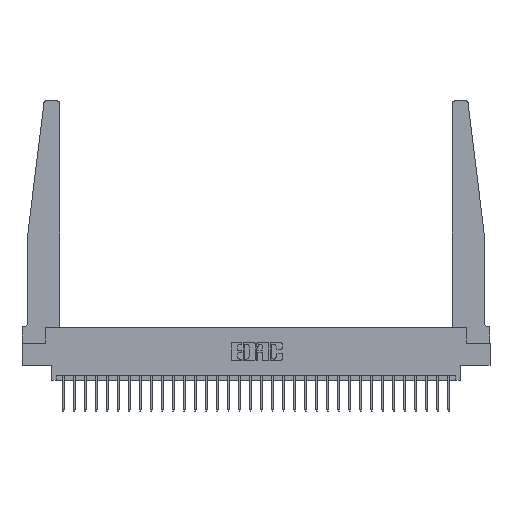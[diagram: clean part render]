
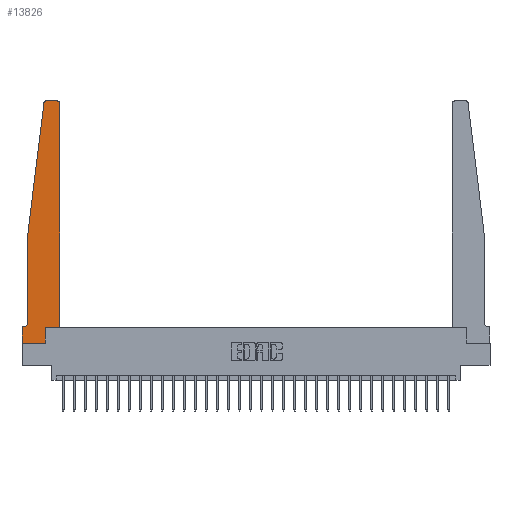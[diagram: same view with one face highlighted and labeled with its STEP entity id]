
A CAD part, top view. The second image highlights one B-rep face of the part: STEP entity #13826.
In plain terms, the highlighted planar face has unit normal (0, 0, 1).
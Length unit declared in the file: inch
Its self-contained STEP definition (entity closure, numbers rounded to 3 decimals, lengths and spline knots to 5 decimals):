
#43 = CARTESIAN_POINT ( 'NONE',  ( 0.015, 0.2375, 0.37 ) ) ;
#174 = EDGE_CURVE ( 'NONE', #27736, #17685, #9732, .T. ) ;
#345 = VERTEX_POINT ( 'NONE', #6715 ) ;
#693 = VECTOR ( 'NONE', #21481, 39.37008 ) ;
#842 = LINE ( 'NONE', #26395, #9476 ) ;
#1305 = DIRECTION ( 'NONE',  ( 0., -1., 0. ) ) ;
#1378 = LINE ( 'NONE', #19375, #19688 ) ;
#1739 = CARTESIAN_POINT ( 'NONE',  ( 0.2605, 0.18, 0.37 ) ) ;
#2248 = VECTOR ( 'NONE', #2393, 39.37008 ) ;
#2262 = CARTESIAN_POINT ( 'NONE',  ( 0.425, 2.72, 0.37 ) ) ;
#2393 = DIRECTION ( 'NONE',  ( -1., 0., 0. ) ) ;
#2428 = DIRECTION ( 'NONE',  ( 0., 0., 1. ) ) ;
#2440 = EDGE_CURVE ( 'NONE', #24999, #11782, #12501, .T. ) ;
#2450 = DIRECTION ( 'NONE',  ( 0., 0., -1. ) ) ;
#2917 = CARTESIAN_POINT ( 'NONE',  ( 0., 0., 0.37 ) ) ;
#2956 = CARTESIAN_POINT ( 'NONE',  ( 0.425, 0.18, 0.37 ) ) ;
#3341 = VECTOR ( 'NONE', #8523, 39.37008 ) ;
#3510 = ORIENTED_EDGE ( 'NONE', *, *, #15467, .T. ) ;
#3787 = CIRCLE ( 'NONE', #24889, 0.03 ) ;
#3964 = EDGE_CURVE ( 'NONE', #28676, #23042, #842, .T. ) ;
#4210 = VERTEX_POINT ( 'NONE', #26830 ) ;
#4221 = VECTOR ( 'NONE', #25952, 39.37008 ) ;
#5036 = DIRECTION ( 'NONE',  ( 0., 1., 0. ) ) ;
#5210 = VERTEX_POINT ( 'NONE', #2956 ) ;
#6071 = ORIENTED_EDGE ( 'NONE', *, *, #174, .T. ) ;
#6579 = ORIENTED_EDGE ( 'NONE', *, *, #21604, .T. ) ;
#6715 = CARTESIAN_POINT ( 'NONE',  ( 0.015, 0.1875, 0.37 ) ) ;
#6956 = DIRECTION ( 'NONE',  ( 1., 0., 0. ) ) ;
#7099 = CARTESIAN_POINT ( 'NONE',  ( 0.065, 1.25, 0.37 ) ) ;
#7100 = EDGE_CURVE ( 'NONE', #17685, #345, #13301, .T. ) ;
#7302 = LINE ( 'NONE', #11934, #28595 ) ;
#7676 = AXIS2_PLACEMENT_3D ( 'NONE', #15869, #11380, #27740 ) ;
#7705 = DIRECTION ( 'NONE',  ( -0.122, -0.992, 0. ) ) ;
#8377 = CIRCLE ( 'NONE', #25133, 0.03 ) ;
#8523 = DIRECTION ( 'NONE',  ( 0., 1., 0. ) ) ;
#8682 = CARTESIAN_POINT ( 'NONE',  ( 0., 0., 0.37 ) ) ;
#8793 = VERTEX_POINT ( 'NONE', #2262 ) ;
#8892 = CARTESIAN_POINT ( 'NONE',  ( 0.065, 0.1875, 0.37 ) ) ;
#9236 = DIRECTION ( 'NONE',  ( -1., 0., 0. ) ) ;
#9476 = VECTOR ( 'NONE', #15243, 39.37008 ) ;
#9732 = LINE ( 'NONE', #14360, #4221 ) ;
#11121 = LINE ( 'NONE', #8892, #2248 ) ;
#11299 = CARTESIAN_POINT ( 'NONE',  ( 0.27653, 2.75, 0.37 ) ) ;
#11380 = DIRECTION ( 'NONE',  ( 0., 0., 1. ) ) ;
#11462 = ORIENTED_EDGE ( 'NONE', *, *, #3964, .T. ) ;
#11782 = VERTEX_POINT ( 'NONE', #11299 ) ;
#11934 = CARTESIAN_POINT ( 'NONE',  ( 0.425, 0.18, 0.37 ) ) ;
#12452 = ORIENTED_EDGE ( 'NONE', *, *, #17511, .T. ) ;
#12501 = LINE ( 'NONE', #21641, #693 ) ;
#13007 = EDGE_CURVE ( 'NONE', #8793, #24999, #3787, .T. ) ;
#13301 = CIRCLE ( 'NONE', #15695, 0.05 ) ;
#13826 = ADVANCED_FACE ( 'NONE', ( #22309 ), #15719, .T. ) ;
#13921 = DIRECTION ( 'NONE',  ( 1., 0., 0. ) ) ;
#14201 = DIRECTION ( 'NONE',  ( 0., 0., 1. ) ) ;
#14360 = CARTESIAN_POINT ( 'NONE',  ( 0.065, 1.25, 0.37 ) ) ;
#15243 = DIRECTION ( 'NONE',  ( 1., 0., 0. ) ) ;
#15252 = LINE ( 'NONE', #8682, #27907 ) ;
#15467 = EDGE_CURVE ( 'NONE', #23042, #4210, #22425, .T. ) ;
#15695 = AXIS2_PLACEMENT_3D ( 'NONE', #43, #2450, #9236 ) ;
#15719 = PLANE ( 'NONE',  #7676 ) ;
#15869 = CARTESIAN_POINT ( 'NONE',  ( 0., 0.1875, 0.37 ) ) ;
#15936 = CARTESIAN_POINT ( 'NONE',  ( 0.395, 2.72, 0.37 ) ) ;
#16184 = EDGE_LOOP ( 'NONE', ( #16270, #6579, #12452, #6071, #29315, #24080, #24011, #11462, #3510, #28584, #24739, #20126 ) ) ;
#16270 = ORIENTED_EDGE ( 'NONE', *, *, #2440, .T. ) ;
#17369 = CARTESIAN_POINT ( 'NONE',  ( 0.395, 2.75, 0.37 ) ) ;
#17511 = EDGE_CURVE ( 'NONE', #19457, #27736, #1378, .T. ) ;
#17685 = VERTEX_POINT ( 'NONE', #22505 ) ;
#17970 = LINE ( 'NONE', #29551, #23192 ) ;
#18494 = EDGE_CURVE ( 'NONE', #29500, #28676, #15252, .T. ) ;
#19375 = CARTESIAN_POINT ( 'NONE',  ( 0.065, 1.25, 0.37 ) ) ;
#19457 = VERTEX_POINT ( 'NONE', #29604 ) ;
#19688 = VECTOR ( 'NONE', #7705, 39.37008 ) ;
#20126 = ORIENTED_EDGE ( 'NONE', *, *, #13007, .T. ) ;
#21481 = DIRECTION ( 'NONE',  ( -1., 0., 0. ) ) ;
#21545 = CARTESIAN_POINT ( 'NONE',  ( 0.27653, 2.72, 0.37 ) ) ;
#21552 = EDGE_CURVE ( 'NONE', #4210, #5210, #17970, .T. ) ;
#21604 = EDGE_CURVE ( 'NONE', #11782, #19457, #8377, .T. ) ;
#21641 = CARTESIAN_POINT ( 'NONE',  ( 0.25, 2.75, 0.37 ) ) ;
#22309 = FACE_OUTER_BOUND ( 'NONE', #16184, .T. ) ;
#22425 = LINE ( 'NONE', #1739, #3341 ) ;
#22505 = CARTESIAN_POINT ( 'NONE',  ( 0.065, 0.2375, 0.37 ) ) ;
#23001 = CARTESIAN_POINT ( 'NONE',  ( 0.2605, 0., 0.37 ) ) ;
#23042 = VERTEX_POINT ( 'NONE', #23001 ) ;
#23192 = VECTOR ( 'NONE', #13921, 39.37008 ) ;
#23240 = CARTESIAN_POINT ( 'NONE',  ( 0., 0.1875, 0.37 ) ) ;
#24011 = ORIENTED_EDGE ( 'NONE', *, *, #18494, .T. ) ;
#24080 = ORIENTED_EDGE ( 'NONE', *, *, #29420, .T. ) ;
#24739 = ORIENTED_EDGE ( 'NONE', *, *, #28631, .T. ) ;
#24889 = AXIS2_PLACEMENT_3D ( 'NONE', #15936, #2428, #6956 ) ;
#24999 = VERTEX_POINT ( 'NONE', #17369 ) ;
#25133 = AXIS2_PLACEMENT_3D ( 'NONE', #21545, #14201, #28031 ) ;
#25952 = DIRECTION ( 'NONE',  ( 0., -1., 0. ) ) ;
#26395 = CARTESIAN_POINT ( 'NONE',  ( 0., 0., 0.37 ) ) ;
#26830 = CARTESIAN_POINT ( 'NONE',  ( 0.2605, 0.18, 0.37 ) ) ;
#27736 = VERTEX_POINT ( 'NONE', #7099 ) ;
#27740 = DIRECTION ( 'NONE',  ( 1., 0., 0. ) ) ;
#27907 = VECTOR ( 'NONE', #1305, 39.37008 ) ;
#28031 = DIRECTION ( 'NONE',  ( 1., 0., 0. ) ) ;
#28584 = ORIENTED_EDGE ( 'NONE', *, *, #21552, .T. ) ;
#28595 = VECTOR ( 'NONE', #5036, 39.37008 ) ;
#28631 = EDGE_CURVE ( 'NONE', #5210, #8793, #7302, .T. ) ;
#28676 = VERTEX_POINT ( 'NONE', #2917 ) ;
#29315 = ORIENTED_EDGE ( 'NONE', *, *, #7100, .T. ) ;
#29420 = EDGE_CURVE ( 'NONE', #345, #29500, #11121, .T. ) ;
#29500 = VERTEX_POINT ( 'NONE', #23240 ) ;
#29551 = CARTESIAN_POINT ( 'NONE',  ( 0.425, 0.18, 0.37 ) ) ;
#29604 = CARTESIAN_POINT ( 'NONE',  ( 0.24675, 2.72367, 0.37 ) ) ;
